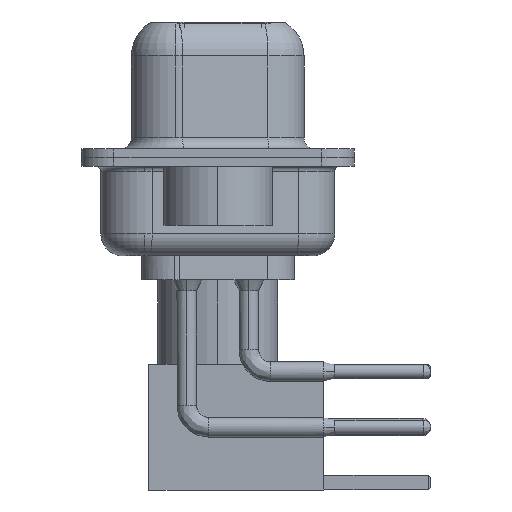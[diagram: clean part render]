
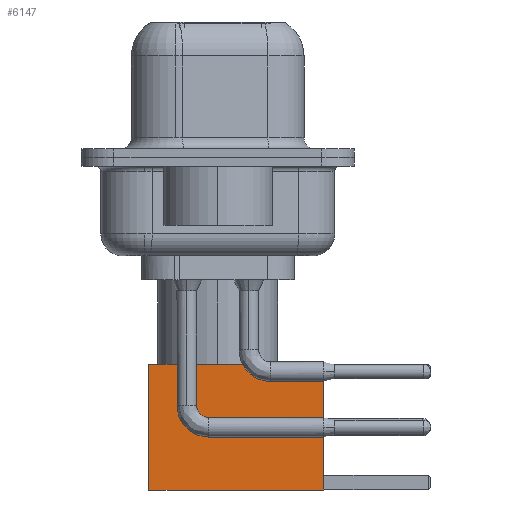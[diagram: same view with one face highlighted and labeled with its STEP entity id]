
A CAD part, left-side view. The second image highlights one B-rep face of the part: STEP entity #6147.
In plain terms, the highlighted face is planar.
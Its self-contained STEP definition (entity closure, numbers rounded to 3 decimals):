
#1524 = FACE_OUTER_BOUND ( 'NONE', #7698, .T. ) ;
#1608 = CARTESIAN_POINT ( 'NONE',  ( 2.875, 2.875, 0. ) ) ;
#2073 = VERTEX_POINT ( 'NONE', #13466 ) ;
#2255 = AXIS2_PLACEMENT_3D ( 'NONE', #15749, #6891, #7004 ) ;
#2686 = CARTESIAN_POINT ( 'NONE',  ( 0., 2.875, 0. ) ) ;
#4100 = VECTOR ( 'NONE', #15172, 1000. ) ;
#4597 = VECTOR ( 'NONE', #6010, 1000. ) ;
#5436 = CARTESIAN_POINT ( 'NONE',  ( 2.875, 2.875, 0. ) ) ;
#6010 = DIRECTION ( 'NONE',  ( 0., 0., -1. ) ) ;
#6095 = EDGE_CURVE ( 'NONE', #9220, #15803, #13886, .T. ) ;
#6147 = ADVANCED_FACE ( 'NONE', ( #1524 ), #22938, .T. ) ;
#6891 = DIRECTION ( 'NONE',  ( 0., 1., 0. ) ) ;
#7004 = DIRECTION ( 'NONE',  ( 0., 0., 1. ) ) ;
#7698 = EDGE_LOOP ( 'NONE', ( #21585, #16661, #9622, #15698 ) ) ;
#9220 = VERTEX_POINT ( 'NONE', #5436 ) ;
#9622 = ORIENTED_EDGE ( 'NONE', *, *, #12747, .F. ) ;
#10411 = LINE ( 'NONE', #20743, #18759 ) ;
#10522 = EDGE_CURVE ( 'NONE', #2073, #9220, #17567, .T. ) ;
#11379 = CARTESIAN_POINT ( 'NONE',  ( -2.875, 2.875, 0. ) ) ;
#12747 = EDGE_CURVE ( 'NONE', #18776, #15803, #22070, .T. ) ;
#13371 = EDGE_CURVE ( 'NONE', #2073, #18776, #10411, .T. ) ;
#13466 = CARTESIAN_POINT ( 'NONE',  ( 2.875, 2.875, 8. ) ) ;
#13886 = LINE ( 'NONE', #2686, #4100 ) ;
#15172 = DIRECTION ( 'NONE',  ( -1., 0., 0. ) ) ;
#15645 = DIRECTION ( 'NONE',  ( -1., 0., 0. ) ) ;
#15698 = ORIENTED_EDGE ( 'NONE', *, *, #13371, .F. ) ;
#15749 = CARTESIAN_POINT ( 'NONE',  ( 2.875, 2.875, 0. ) ) ;
#15803 = VERTEX_POINT ( 'NONE', #16653 ) ;
#16653 = CARTESIAN_POINT ( 'NONE',  ( -2.875, 2.875, 0. ) ) ;
#16661 = ORIENTED_EDGE ( 'NONE', *, *, #6095, .T. ) ;
#17567 = LINE ( 'NONE', #1608, #17985 ) ;
#17985 = VECTOR ( 'NONE', #19531, 1000. ) ;
#18759 = VECTOR ( 'NONE', #15645, 1000. ) ;
#18776 = VERTEX_POINT ( 'NONE', #20147 ) ;
#19531 = DIRECTION ( 'NONE',  ( 0., 0., -1. ) ) ;
#20147 = CARTESIAN_POINT ( 'NONE',  ( -2.875, 2.875, 8. ) ) ;
#20743 = CARTESIAN_POINT ( 'NONE',  ( 0., 2.875, 8. ) ) ;
#21585 = ORIENTED_EDGE ( 'NONE', *, *, #10522, .T. ) ;
#22070 = LINE ( 'NONE', #11379, #4597 ) ;
#22938 = PLANE ( 'NONE',  #2255 ) ;
